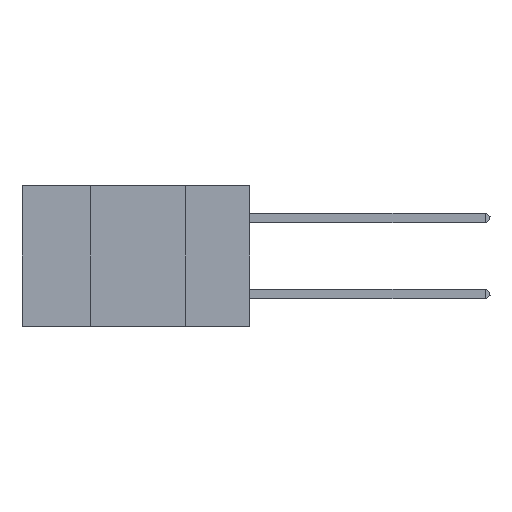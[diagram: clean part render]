
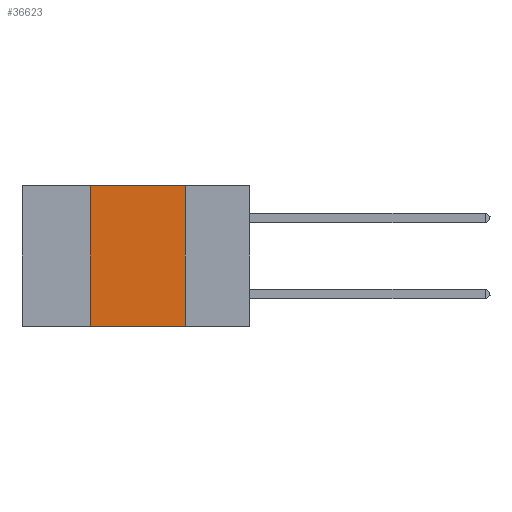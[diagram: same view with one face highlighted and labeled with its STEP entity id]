
A CAD part, left-side view. The second image highlights one B-rep face of the part: STEP entity #36623.
In plain terms, the highlighted planar face has unit normal (-1, 0, 0).
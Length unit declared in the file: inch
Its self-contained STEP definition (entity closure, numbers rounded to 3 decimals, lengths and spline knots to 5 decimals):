
#924 = VERTEX_POINT ( 'NONE', #44154 ) ;
#3651 = DIRECTION ( 'NONE',  ( 0., 0., -1. ) ) ;
#3804 = VECTOR ( 'NONE', #5844, 39.37008 ) ;
#3974 = EDGE_CURVE ( 'NONE', #28481, #31956, #42891, .T. ) ;
#5844 = DIRECTION ( 'NONE',  ( 0., -1., 0. ) ) ;
#7242 = PLANE ( 'NONE',  #31555 ) ;
#7965 = CARTESIAN_POINT ( 'NONE',  ( 0., 0.17, 0. ) ) ;
#8955 = CARTESIAN_POINT ( 'NONE',  ( 0., 0.6, 0. ) ) ;
#12325 = LINE ( 'NONE', #7965, #39603 ) ;
#13295 = EDGE_CURVE ( 'NONE', #28892, #31956, #12325, .T. ) ;
#13574 = CARTESIAN_POINT ( 'NONE',  ( 0., 0.17, 0. ) ) ;
#14045 = EDGE_LOOP ( 'NONE', ( #24493, #24611, #39779, #15351 ) ) ;
#15351 = ORIENTED_EDGE ( 'NONE', *, *, #3974, .T. ) ;
#17190 = LINE ( 'NONE', #8955, #3804 ) ;
#17607 = FACE_OUTER_BOUND ( 'NONE', #14045, .T. ) ;
#18795 = CARTESIAN_POINT ( 'NONE',  ( 0., 0.6, -0.37 ) ) ;
#19092 = EDGE_CURVE ( 'NONE', #924, #28892, #17190, .T. ) ;
#21601 = DIRECTION ( 'NONE',  ( 1., 0., 0. ) ) ;
#24493 = ORIENTED_EDGE ( 'NONE', *, *, #13295, .F. ) ;
#24611 = ORIENTED_EDGE ( 'NONE', *, *, #19092, .F. ) ;
#25189 = CARTESIAN_POINT ( 'NONE',  ( 0., 0.42, 0. ) ) ;
#26038 = CARTESIAN_POINT ( 'NONE',  ( 0., 0.17, -0.37 ) ) ;
#26169 = VECTOR ( 'NONE', #43696, 39.37008 ) ;
#26940 = LINE ( 'NONE', #25189, #29090 ) ;
#28481 = VERTEX_POINT ( 'NONE', #35266 ) ;
#28892 = VERTEX_POINT ( 'NONE', #13574 ) ;
#29090 = VECTOR ( 'NONE', #42634, 39.37008 ) ;
#31555 = AXIS2_PLACEMENT_3D ( 'NONE', #31691, #21601, #3651 ) ;
#31691 = CARTESIAN_POINT ( 'NONE',  ( 0., 0.6, 0. ) ) ;
#31956 = VERTEX_POINT ( 'NONE', #26038 ) ;
#32452 = EDGE_CURVE ( 'NONE', #28481, #924, #26940, .T. ) ;
#32889 = DIRECTION ( 'NONE',  ( 0., 0., -1. ) ) ;
#35266 = CARTESIAN_POINT ( 'NONE',  ( 0., 0.42, -0.37 ) ) ;
#36623 = ADVANCED_FACE ( 'NONE', ( #17607 ), #7242, .F. ) ;
#39603 = VECTOR ( 'NONE', #32889, 39.37008 ) ;
#39779 = ORIENTED_EDGE ( 'NONE', *, *, #32452, .F. ) ;
#42634 = DIRECTION ( 'NONE',  ( 0., 0., 1. ) ) ;
#42891 = LINE ( 'NONE', #18795, #26169 ) ;
#43696 = DIRECTION ( 'NONE',  ( 0., -1., 0. ) ) ;
#44154 = CARTESIAN_POINT ( 'NONE',  ( 0., 0.42, 0. ) ) ;
